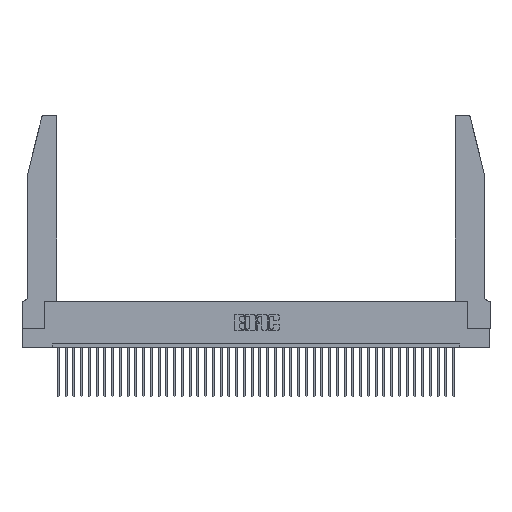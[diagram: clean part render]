
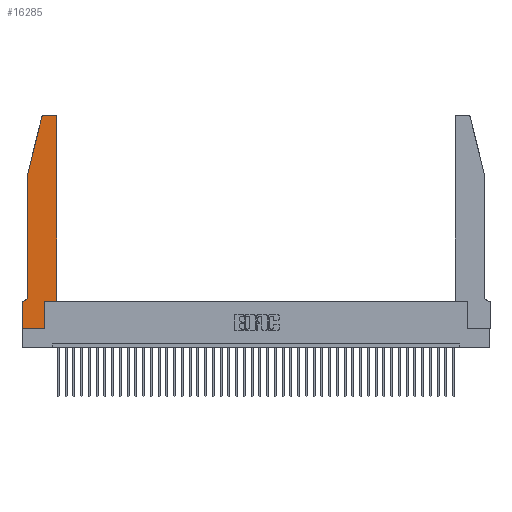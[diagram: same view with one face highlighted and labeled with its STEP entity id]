
A CAD part, top view. The second image highlights one B-rep face of the part: STEP entity #16285.
In plain terms, the highlighted planar face has unit normal (0, 0, 1).
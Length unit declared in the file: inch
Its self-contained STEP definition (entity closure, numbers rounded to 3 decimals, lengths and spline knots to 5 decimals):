
#496 = DIRECTION ( 'NONE',  ( 0., 1., 0. ) ) ;
#587 = DIRECTION ( 'NONE',  ( 0., -1., 0. ) ) ;
#740 = CIRCLE ( 'NONE', #19959, 0.03 ) ;
#959 = CIRCLE ( 'NONE', #38820, 0.07 ) ;
#1308 = VERTEX_POINT ( 'NONE', #30952 ) ;
#1870 = EDGE_CURVE ( 'NONE', #16604, #40975, #39598, .T. ) ;
#3098 = VECTOR ( 'NONE', #13824, 39.37008 ) ;
#3179 = VECTOR ( 'NONE', #496, 39.37008 ) ;
#3502 = LINE ( 'NONE', #32332, #29696 ) ;
#4220 = VERTEX_POINT ( 'NONE', #7247 ) ;
#4786 = VERTEX_POINT ( 'NONE', #40666 ) ;
#5349 = VECTOR ( 'NONE', #20630, 39.37008 ) ;
#5461 = EDGE_LOOP ( 'NONE', ( #19323, #37627, #13919, #15860, #31272, #18872, #9516, #24790, #30822, #41602, #21934, #18993 ) ) ;
#5616 = AXIS2_PLACEMENT_3D ( 'NONE', #26975, #20640, #10276 ) ;
#6371 = LINE ( 'NONE', #23654, #5349 ) ;
#6576 = DIRECTION ( 'NONE',  ( 1., 0., 0. ) ) ;
#6718 = CARTESIAN_POINT ( 'NONE',  ( 0.4505, 0.35, 0.37 ) ) ;
#7247 = CARTESIAN_POINT ( 'NONE',  ( 0.0055, 0.35, 0.37 ) ) ;
#7739 = CARTESIAN_POINT ( 'NONE',  ( 0., 0.35, 0.37 ) ) ;
#8012 = VERTEX_POINT ( 'NONE', #41231 ) ;
#8183 = LINE ( 'NONE', #6718, #20079 ) ;
#9516 = ORIENTED_EDGE ( 'NONE', *, *, #1870, .T. ) ;
#9993 = DIRECTION ( 'NONE',  ( 0., 0., -1. ) ) ;
#10233 = CARTESIAN_POINT ( 'NONE',  ( 0.2865, 0.35, 0.37 ) ) ;
#10276 = DIRECTION ( 'NONE',  ( 1., 0., 0. ) ) ;
#10294 = VERTEX_POINT ( 'NONE', #30789 ) ;
#10335 = CARTESIAN_POINT ( 'NONE',  ( 0.2865, 0.35, 0.37 ) ) ;
#11065 = PLANE ( 'NONE',  #30108 ) ;
#11410 = CARTESIAN_POINT ( 'NONE',  ( 0.4505, 0.35, 0.37 ) ) ;
#12173 = EDGE_CURVE ( 'NONE', #8012, #4220, #959, .T. ) ;
#13349 = VECTOR ( 'NONE', #26990, 39.37008 ) ;
#13471 = VECTOR ( 'NONE', #15669, 39.37008 ) ;
#13776 = CARTESIAN_POINT ( 'NONE',  ( 0.4205, 2.72, 0.37 ) ) ;
#13824 = DIRECTION ( 'NONE',  ( 0., -1., 0. ) ) ;
#13919 = ORIENTED_EDGE ( 'NONE', *, *, #29354, .T. ) ;
#14043 = VECTOR ( 'NONE', #38782, 39.37008 ) ;
#14630 = FACE_OUTER_BOUND ( 'NONE', #5461, .T. ) ;
#14742 = CIRCLE ( 'NONE', #5616, 0.03 ) ;
#15669 = DIRECTION ( 'NONE',  ( -1., 0., 0. ) ) ;
#15860 = ORIENTED_EDGE ( 'NONE', *, *, #19601, .T. ) ;
#16285 = ADVANCED_FACE ( 'NONE', ( #14630 ), #11065, .T. ) ;
#16518 = LINE ( 'NONE', #41340, #14043 ) ;
#16592 = VECTOR ( 'NONE', #19991, 39.37008 ) ;
#16604 = VERTEX_POINT ( 'NONE', #22425 ) ;
#16701 = EDGE_CURVE ( 'NONE', #4220, #16604, #39686, .T. ) ;
#16965 = CARTESIAN_POINT ( 'NONE',  ( 0., 0., 0.37 ) ) ;
#17936 = CARTESIAN_POINT ( 'NONE',  ( 0.2865, 0., 0.37 ) ) ;
#18872 = ORIENTED_EDGE ( 'NONE', *, *, #16701, .T. ) ;
#18993 = ORIENTED_EDGE ( 'NONE', *, *, #21552, .T. ) ;
#19107 = CARTESIAN_POINT ( 'NONE',  ( 0.0755, 0.35, 0.37 ) ) ;
#19323 = ORIENTED_EDGE ( 'NONE', *, *, #37552, .T. ) ;
#19601 = EDGE_CURVE ( 'NONE', #40642, #8012, #3502, .T. ) ;
#19959 = AXIS2_PLACEMENT_3D ( 'NONE', #13776, #29857, #20383 ) ;
#19991 = DIRECTION ( 'NONE',  ( 0., 1., 0. ) ) ;
#20079 = VECTOR ( 'NONE', #6576, 39.37008 ) ;
#20180 = VERTEX_POINT ( 'NONE', #25703 ) ;
#20374 = EDGE_CURVE ( 'NONE', #10294, #20180, #14742, .T. ) ;
#20383 = DIRECTION ( 'NONE',  ( 1., 0., 0. ) ) ;
#20630 = DIRECTION ( 'NONE',  ( 1., 0., 0. ) ) ;
#20640 = DIRECTION ( 'NONE',  ( 0., 0., 1. ) ) ;
#20655 = LINE ( 'NONE', #10233, #3179 ) ;
#20723 = DIRECTION ( 'NONE',  ( 1., 0., 0. ) ) ;
#21552 = EDGE_CURVE ( 'NONE', #1308, #4786, #740, .T. ) ;
#21934 = ORIENTED_EDGE ( 'NONE', *, *, #26224, .T. ) ;
#22095 = LINE ( 'NONE', #23531, #13349 ) ;
#22425 = CARTESIAN_POINT ( 'NONE',  ( 0., 0.35, 0.37 ) ) ;
#23531 = CARTESIAN_POINT ( 'NONE',  ( 0.0755, 2., 0.37 ) ) ;
#23654 = CARTESIAN_POINT ( 'NONE',  ( 0., 0., 0.37 ) ) ;
#24296 = DIRECTION ( 'NONE',  ( 0., 0., 1. ) ) ;
#24790 = ORIENTED_EDGE ( 'NONE', *, *, #36114, .T. ) ;
#25703 = CARTESIAN_POINT ( 'NONE',  ( 0.25487, 2.72718, 0.37 ) ) ;
#26137 = CARTESIAN_POINT ( 'NONE',  ( 0.0055, 0.42, 0.37 ) ) ;
#26224 = EDGE_CURVE ( 'NONE', #33598, #1308, #32003, .T. ) ;
#26975 = CARTESIAN_POINT ( 'NONE',  ( 0.284, 2.72, 0.37 ) ) ;
#26990 = DIRECTION ( 'NONE',  ( -0.239, -0.971, 0. ) ) ;
#29354 = EDGE_CURVE ( 'NONE', #20180, #40642, #22095, .T. ) ;
#29413 = DIRECTION ( 'NONE',  ( -1., 0., 0. ) ) ;
#29696 = VECTOR ( 'NONE', #587, 39.37008 ) ;
#29857 = DIRECTION ( 'NONE',  ( 0., 0., 1. ) ) ;
#30108 = AXIS2_PLACEMENT_3D ( 'NONE', #7739, #24296, #20723 ) ;
#30789 = CARTESIAN_POINT ( 'NONE',  ( 0.284, 2.75, 0.37 ) ) ;
#30822 = ORIENTED_EDGE ( 'NONE', *, *, #41641, .T. ) ;
#30952 = CARTESIAN_POINT ( 'NONE',  ( 0.4505, 2.72, 0.37 ) ) ;
#31272 = ORIENTED_EDGE ( 'NONE', *, *, #12173, .T. ) ;
#32003 = LINE ( 'NONE', #33470, #16592 ) ;
#32150 = CARTESIAN_POINT ( 'NONE',  ( 0., 0., 0.37 ) ) ;
#32332 = CARTESIAN_POINT ( 'NONE',  ( 0.0755, 2., 0.37 ) ) ;
#33470 = CARTESIAN_POINT ( 'NONE',  ( 0.4505, 0.35, 0.37 ) ) ;
#33598 = VERTEX_POINT ( 'NONE', #11410 ) ;
#34307 = CARTESIAN_POINT ( 'NONE',  ( 0.0755, 2., 0.37 ) ) ;
#34889 = EDGE_CURVE ( 'NONE', #40566, #33598, #8183, .T. ) ;
#36114 = EDGE_CURVE ( 'NONE', #40975, #40786, #6371, .T. ) ;
#37552 = EDGE_CURVE ( 'NONE', #4786, #10294, #16518, .T. ) ;
#37627 = ORIENTED_EDGE ( 'NONE', *, *, #20374, .T. ) ;
#38782 = DIRECTION ( 'NONE',  ( -1., 0., 0. ) ) ;
#38820 = AXIS2_PLACEMENT_3D ( 'NONE', #26137, #9993, #29413 ) ;
#39598 = LINE ( 'NONE', #16965, #3098 ) ;
#39686 = LINE ( 'NONE', #19107, #13471 ) ;
#40566 = VERTEX_POINT ( 'NONE', #10335 ) ;
#40642 = VERTEX_POINT ( 'NONE', #34307 ) ;
#40666 = CARTESIAN_POINT ( 'NONE',  ( 0.4205, 2.75, 0.37 ) ) ;
#40786 = VERTEX_POINT ( 'NONE', #17936 ) ;
#40975 = VERTEX_POINT ( 'NONE', #32150 ) ;
#41231 = CARTESIAN_POINT ( 'NONE',  ( 0.0755, 0.42, 0.37 ) ) ;
#41340 = CARTESIAN_POINT ( 'NONE',  ( 0.2605, 2.75, 0.37 ) ) ;
#41602 = ORIENTED_EDGE ( 'NONE', *, *, #34889, .T. ) ;
#41641 = EDGE_CURVE ( 'NONE', #40786, #40566, #20655, .T. ) ;
